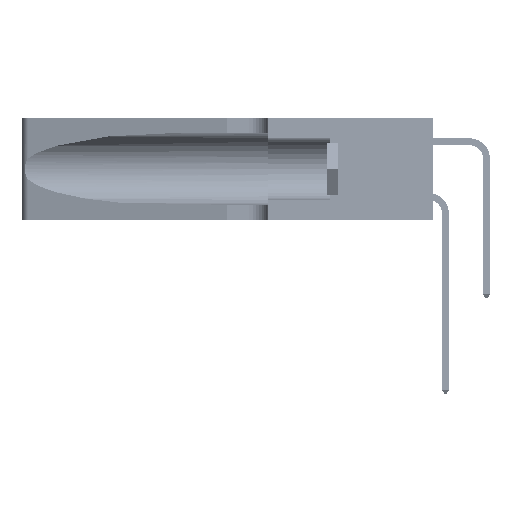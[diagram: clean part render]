
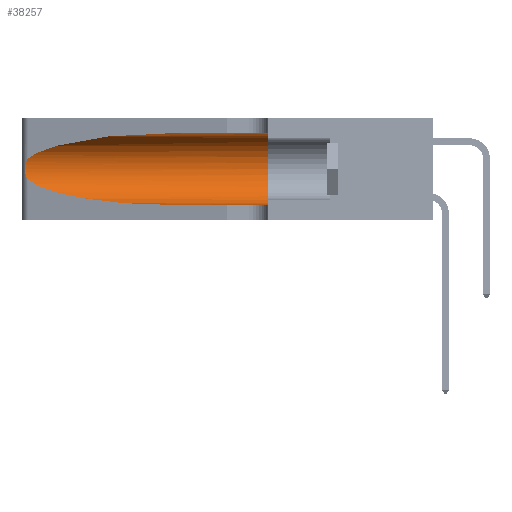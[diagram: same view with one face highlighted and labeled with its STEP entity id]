
A CAD part, left-side view. The second image highlights one B-rep face of the part: STEP entity #38257.
In plain terms, the highlighted cylindrical face has radius 3.308 mm (diameter 6.617 mm), a partial arc.
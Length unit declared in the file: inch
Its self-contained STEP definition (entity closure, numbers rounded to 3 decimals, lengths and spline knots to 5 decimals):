
#3477 = CARTESIAN_POINT ( 'NONE',  ( 0.25487, 1.22718, 0.14631 ) ) ;
#3839 = CARTESIAN_POINT ( 'NONE',  ( 0.26018, 1.23835, 0.19895 ) ) ;
#4250 = VERTEX_POINT ( 'NONE', #33683 ) ;
#4269 = CARTESIAN_POINT ( 'NONE',  ( 0.1305, 0.35, 0.05475 ) ) ;
#4344 =( BOUNDED_CURVE ( )  B_SPLINE_CURVE ( 3, ( #3477, #27882, #35939, #11764 ),
 .UNSPECIFIED., .F., .T. ) 
 B_SPLINE_CURVE_WITH_KNOTS ( ( 4, 4 ),
 ( 3.44316, 4.71239 ),
 .UNSPECIFIED. ) 
 CURVE ( )  GEOMETRIC_REPRESENTATION_ITEM ( )  RATIONAL_B_SPLINE_CURVE ( ( 1., 0.87, 0.87, 1. ) ) 
 REPRESENTATION_ITEM ( '' )  );
#6003 =( BOUNDED_CURVE ( )  B_SPLINE_CURVE ( 3, ( #27269, #35360, #15250, #43347 ),
 .UNSPECIFIED., .F., .F. ) 
 B_SPLINE_CURVE_WITH_KNOTS ( ( 4, 4 ),
 ( 1.5708, 2.84003 ),
 .UNSPECIFIED. ) 
 CURVE ( )  GEOMETRIC_REPRESENTATION_ITEM ( )  RATIONAL_B_SPLINE_CURVE ( ( 1., 0.87, 0.87, 1. ) ) 
 REPRESENTATION_ITEM ( '' )  );
#7982 = CARTESIAN_POINT ( 'NONE',  ( 0.26075, 1.23896, 0.178 ) ) ;
#8609 = LINE ( 'NONE', #38828, #48903 ) ;
#10166 = CARTESIAN_POINT ( 'NONE',  ( 0.1305, 1.61858, 0.185 ) ) ;
#11080 = AXIS2_PLACEMENT_3D ( 'NONE', #10166, #38391, #34408 ) ;
#11240 = LINE ( 'NONE', #48979, #20777 ) ;
#11340 = CARTESIAN_POINT ( 'NONE',  ( 0.1305, 0.35, 0.185 ) ) ;
#11447 = CARTESIAN_POINT ( 'NONE',  ( 0.25487, 1.22718, 0.22369 ) ) ;
#11764 = CARTESIAN_POINT ( 'NONE',  ( 0.1305, 0.72297, 0.05475 ) ) ;
#11942 = CARTESIAN_POINT ( 'NONE',  ( 0.25487, 1.22718, 0.22369 ) ) ;
#12124 = CARTESIAN_POINT ( 'NONE',  ( 0.25856, 1.23593, 0.16098 ) ) ;
#12555 = VERTEX_POINT ( 'NONE', #26299 ) ;
#15250 = CARTESIAN_POINT ( 'NONE',  ( 0.2373, 1.15595, 0.28018 ) ) ;
#15402 = EDGE_CURVE ( 'NONE', #4250, #37960, #8609, .T. ) ;
#15442 = DIRECTION ( 'NONE',  ( 0., 0., 1. ) ) ;
#16214 = CARTESIAN_POINT ( 'NONE',  ( 0.25639, 1.23186, 0.15144 ) ) ;
#16769 = FACE_OUTER_BOUND ( 'NONE', #46358, .T. ) ;
#20293 = CARTESIAN_POINT ( 'NONE',  ( 0.25487, 1.22718, 0.14631 ) ) ;
#20777 = VECTOR ( 'NONE', #49149, 39.37008 ) ;
#24166 = CARTESIAN_POINT ( 'NONE',  ( 0.25639, 1.23184, 0.21858 ) ) ;
#24924 = B_SPLINE_CURVE_WITH_KNOTS ( 'NONE', 3,
 ( #11942, #36116, #24166, #52110, #28237, #3839, #32282, #7982, #36282, #12124, #40270, #16214, #44302, #20293 ),
 .UNSPECIFIED., .F., .F.,
 ( 4, 2, 2, 2, 2, 2, 4 ),
 ( 0., 0.00027, 0.00053, 0.00107, 0.0016, 0.00187, 0.00214 ),
 .UNSPECIFIED. ) ;
#25080 = CIRCLE ( 'NONE', #27219, 0.13025 ) ;
#26299 = CARTESIAN_POINT ( 'NONE',  ( 0.1305, 0.72297, 0.31525 ) ) ;
#26756 = DIRECTION ( 'NONE',  ( 0., -1., 0. ) ) ;
#27219 = AXIS2_PLACEMENT_3D ( 'NONE', #11340, #39526, #15442 ) ;
#27269 = CARTESIAN_POINT ( 'NONE',  ( 0.1305, 0.72297, 0.31525 ) ) ;
#27493 = EDGE_CURVE ( 'NONE', #43079, #4250, #4344, .T. ) ;
#27725 = EDGE_CURVE ( 'NONE', #12555, #47448, #11240, .T. ) ;
#27882 = CARTESIAN_POINT ( 'NONE',  ( 0.2373, 1.15595, 0.08982 ) ) ;
#28237 = CARTESIAN_POINT ( 'NONE',  ( 0.25854, 1.2359, 0.20912 ) ) ;
#29773 = VERTEX_POINT ( 'NONE', #11447 ) ;
#29863 = CARTESIAN_POINT ( 'NONE',  ( 0.1305, 0.35, 0.31525 ) ) ;
#32282 = CARTESIAN_POINT ( 'NONE',  ( 0.26075, 1.23896, 0.19203 ) ) ;
#33339 = EDGE_CURVE ( 'NONE', #47448, #37960, #25080, .T. ) ;
#33683 = CARTESIAN_POINT ( 'NONE',  ( 0.1305, 0.72297, 0.05475 ) ) ;
#34408 = DIRECTION ( 'NONE',  ( 0., 0., -1. ) ) ;
#35304 = ORIENTED_EDGE ( 'NONE', *, *, #33339, .F. ) ;
#35360 = CARTESIAN_POINT ( 'NONE',  ( 0.18966, 0.96281, 0.31525 ) ) ;
#35939 = CARTESIAN_POINT ( 'NONE',  ( 0.18966, 0.96281, 0.05475 ) ) ;
#36116 = CARTESIAN_POINT ( 'NONE',  ( 0.25555, 1.22994, 0.2215 ) ) ;
#36282 = CARTESIAN_POINT ( 'NONE',  ( 0.26017, 1.23833, 0.17102 ) ) ;
#37960 = VERTEX_POINT ( 'NONE', #4269 ) ;
#38257 = ADVANCED_FACE ( 'NONE', ( #16769 ), #46292, .F. ) ;
#38391 = DIRECTION ( 'NONE',  ( 0., -1., 0. ) ) ;
#38471 = CARTESIAN_POINT ( 'NONE',  ( 0.25487, 1.22718, 0.14631 ) ) ;
#38828 = CARTESIAN_POINT ( 'NONE',  ( 0.1305, 1.61858, 0.05475 ) ) ;
#39526 = DIRECTION ( 'NONE',  ( 0., 1., 0. ) ) ;
#39542 = ORIENTED_EDGE ( 'NONE', *, *, #15402, .T. ) ;
#40270 = CARTESIAN_POINT ( 'NONE',  ( 0.25789, 1.23486, 0.15765 ) ) ;
#42897 = ORIENTED_EDGE ( 'NONE', *, *, #44560, .T. ) ;
#43079 = VERTEX_POINT ( 'NONE', #38471 ) ;
#43347 = CARTESIAN_POINT ( 'NONE',  ( 0.25487, 1.22718, 0.22369 ) ) ;
#44302 = CARTESIAN_POINT ( 'NONE',  ( 0.25555, 1.22993, 0.14849 ) ) ;
#44560 = EDGE_CURVE ( 'NONE', #29773, #43079, #24924, .T. ) ;
#46292 = CYLINDRICAL_SURFACE ( 'NONE', #11080, 0.13025 ) ;
#46358 = EDGE_LOOP ( 'NONE', ( #51416, #42897, #50483, #39542, #35304, #47875 ) ) ;
#47020 = EDGE_CURVE ( 'NONE', #12555, #29773, #6003, .T. ) ;
#47448 = VERTEX_POINT ( 'NONE', #29863 ) ;
#47875 = ORIENTED_EDGE ( 'NONE', *, *, #27725, .F. ) ;
#48903 = VECTOR ( 'NONE', #26756, 39.37008 ) ;
#48979 = CARTESIAN_POINT ( 'NONE',  ( 0.1305, 1.61858, 0.31525 ) ) ;
#49149 = DIRECTION ( 'NONE',  ( 0., -1., 0. ) ) ;
#50483 = ORIENTED_EDGE ( 'NONE', *, *, #27493, .T. ) ;
#51416 = ORIENTED_EDGE ( 'NONE', *, *, #47020, .T. ) ;
#52110 = CARTESIAN_POINT ( 'NONE',  ( 0.25787, 1.23484, 0.2124 ) ) ;
